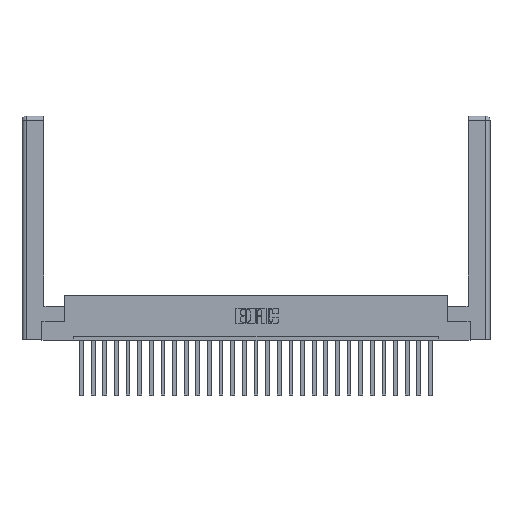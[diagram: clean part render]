
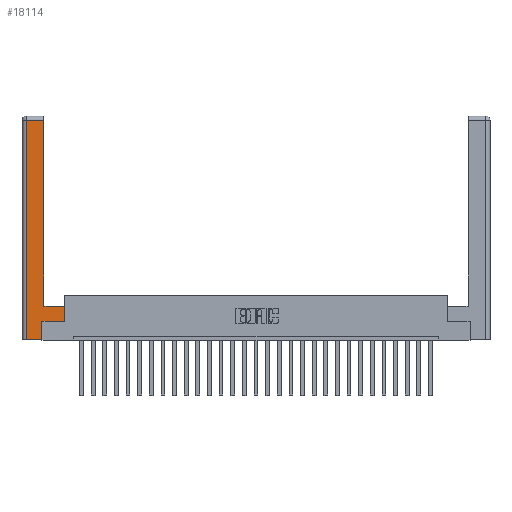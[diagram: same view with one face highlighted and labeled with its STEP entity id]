
A CAD part, top view. The second image highlights one B-rep face of the part: STEP entity #18114.
In plain terms, the highlighted planar face has unit normal (0, 0, 1).
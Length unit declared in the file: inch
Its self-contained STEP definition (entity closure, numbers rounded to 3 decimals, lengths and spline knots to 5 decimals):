
#152 = ORIENTED_EDGE ( 'NONE', *, *, #15010, .T. ) ;
#359 = VERTEX_POINT ( 'NONE', #8921 ) ;
#1349 = EDGE_CURVE ( 'NONE', #6535, #359, #25512, .T. ) ;
#1717 = AXIS2_PLACEMENT_3D ( 'NONE', #17251, #13239, #4792 ) ;
#2059 = DIRECTION ( 'NONE',  ( 0., 1., 0. ) ) ;
#2563 = VECTOR ( 'NONE', #23658, 39.37008 ) ;
#3563 = VERTEX_POINT ( 'NONE', #8249 ) ;
#3895 = CARTESIAN_POINT ( 'NONE',  ( 0.565, 0.45, 0. ) ) ;
#4413 = ORIENTED_EDGE ( 'NONE', *, *, #1349, .T. ) ;
#4577 = CARTESIAN_POINT ( 'NONE',  ( 0.265, 0., 0. ) ) ;
#4655 = LINE ( 'NONE', #24191, #15724 ) ;
#4792 = DIRECTION ( 'NONE',  ( -1., 0., 0. ) ) ;
#6300 = VECTOR ( 'NONE', #24630, 39.37008 ) ;
#6535 = VERTEX_POINT ( 'NONE', #9418 ) ;
#6638 = PLANE ( 'NONE',  #1717 ) ;
#6870 = ORIENTED_EDGE ( 'NONE', *, *, #23476, .T. ) ;
#7297 = CARTESIAN_POINT ( 'NONE',  ( 0.565, 0.245, 0. ) ) ;
#7472 = VECTOR ( 'NONE', #18714, 39.37008 ) ;
#7580 = VECTOR ( 'NONE', #8952, 39.37008 ) ;
#8249 = CARTESIAN_POINT ( 'NONE',  ( 0.295, 0.45, 0. ) ) ;
#8642 = LINE ( 'NONE', #7297, #22584 ) ;
#8921 = CARTESIAN_POINT ( 'NONE',  ( 0.565, 0.45, 0. ) ) ;
#8952 = DIRECTION ( 'NONE',  ( 1., 0., 0. ) ) ;
#9418 = CARTESIAN_POINT ( 'NONE',  ( 0.565, 0.245, 0. ) ) ;
#9991 = CARTESIAN_POINT ( 'NONE',  ( 0.265, 0.245, 0. ) ) ;
#10465 = LINE ( 'NONE', #4577, #7580 ) ;
#10831 = ORIENTED_EDGE ( 'NONE', *, *, #18271, .T. ) ;
#10932 = EDGE_LOOP ( 'NONE', ( #152, #10831, #13377, #6870, #17752, #20130, #4413, #21134 ) ) ;
#11744 = DIRECTION ( 'NONE',  ( 1., 0., 0. ) ) ;
#11846 = FACE_OUTER_BOUND ( 'NONE', #10932, .T. ) ;
#13017 = CARTESIAN_POINT ( 'NONE',  ( 0.265, 0.245, 0. ) ) ;
#13239 = DIRECTION ( 'NONE',  ( 0., 0., -1. ) ) ;
#13377 = ORIENTED_EDGE ( 'NONE', *, *, #25979, .T. ) ;
#13559 = VERTEX_POINT ( 'NONE', #13017 ) ;
#13854 = VECTOR ( 'NONE', #2059, 39.37008 ) ;
#14246 = VERTEX_POINT ( 'NONE', #19397 ) ;
#15010 = EDGE_CURVE ( 'NONE', #3563, #14246, #15227, .T. ) ;
#15227 = LINE ( 'NONE', #25773, #2563 ) ;
#15724 = VECTOR ( 'NONE', #20021, 39.37008 ) ;
#15746 = EDGE_CURVE ( 'NONE', #359, #3563, #19119, .T. ) ;
#15839 = CARTESIAN_POINT ( 'NONE',  ( 0.0615, 0., 0. ) ) ;
#15922 = DIRECTION ( 'NONE',  ( 0., -1., 0. ) ) ;
#16131 = VERTEX_POINT ( 'NONE', #19625 ) ;
#16988 = LINE ( 'NONE', #9991, #6300 ) ;
#17139 = VERTEX_POINT ( 'NONE', #21973 ) ;
#17251 = CARTESIAN_POINT ( 'NONE',  ( 0., 0., 0. ) ) ;
#17752 = ORIENTED_EDGE ( 'NONE', *, *, #18833, .T. ) ;
#18114 = ADVANCED_FACE ( 'NONE', ( #11846 ), #6638, .F. ) ;
#18250 = VERTEX_POINT ( 'NONE', #20286 ) ;
#18271 = EDGE_CURVE ( 'NONE', #14246, #16131, #4655, .T. ) ;
#18714 = DIRECTION ( 'NONE',  ( -1., 0., 0. ) ) ;
#18833 = EDGE_CURVE ( 'NONE', #17139, #13559, #16988, .T. ) ;
#19119 = LINE ( 'NONE', #26891, #7472 ) ;
#19397 = CARTESIAN_POINT ( 'NONE',  ( 0.295, 2.94, 0. ) ) ;
#19625 = CARTESIAN_POINT ( 'NONE',  ( 0.0615, 2.94, 0. ) ) ;
#20021 = DIRECTION ( 'NONE',  ( -1., 0., 0. ) ) ;
#20130 = ORIENTED_EDGE ( 'NONE', *, *, #21759, .T. ) ;
#20286 = CARTESIAN_POINT ( 'NONE',  ( 0.0615, 0., 0. ) ) ;
#21134 = ORIENTED_EDGE ( 'NONE', *, *, #15746, .T. ) ;
#21759 = EDGE_CURVE ( 'NONE', #13559, #6535, #8642, .T. ) ;
#21973 = CARTESIAN_POINT ( 'NONE',  ( 0.265, 0., 0. ) ) ;
#22584 = VECTOR ( 'NONE', #11744, 39.37008 ) ;
#23476 = EDGE_CURVE ( 'NONE', #18250, #17139, #10465, .T. ) ;
#23658 = DIRECTION ( 'NONE',  ( 0., 1., 0. ) ) ;
#24191 = CARTESIAN_POINT ( 'NONE',  ( 0.0615, 2.94, 0. ) ) ;
#24210 = LINE ( 'NONE', #15839, #24513 ) ;
#24513 = VECTOR ( 'NONE', #15922, 39.37008 ) ;
#24630 = DIRECTION ( 'NONE',  ( 0., 1., 0. ) ) ;
#25512 = LINE ( 'NONE', #3895, #13854 ) ;
#25773 = CARTESIAN_POINT ( 'NONE',  ( 0.295, 3., 0. ) ) ;
#25979 = EDGE_CURVE ( 'NONE', #16131, #18250, #24210, .T. ) ;
#26891 = CARTESIAN_POINT ( 'NONE',  ( 0.295, 0.45, 0. ) ) ;
